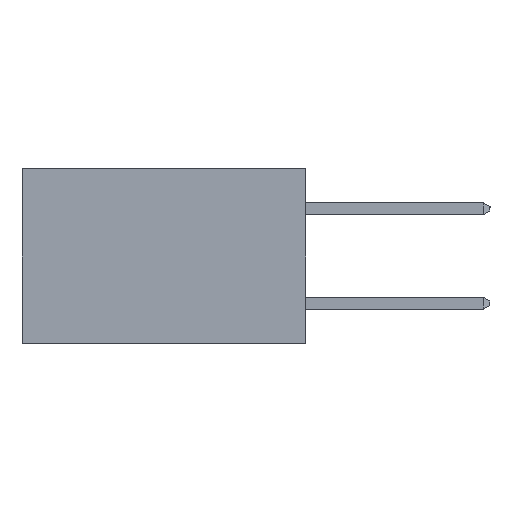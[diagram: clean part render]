
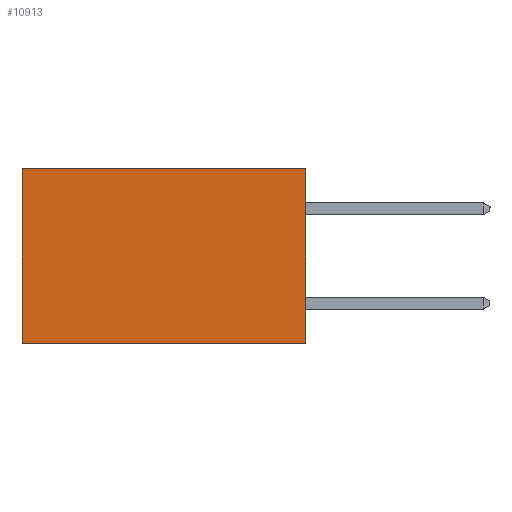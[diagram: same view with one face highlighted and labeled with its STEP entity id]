
A CAD part, left-side view. The second image highlights one B-rep face of the part: STEP entity #10913.
In plain terms, the highlighted planar face has unit normal (-1, 0, 0).
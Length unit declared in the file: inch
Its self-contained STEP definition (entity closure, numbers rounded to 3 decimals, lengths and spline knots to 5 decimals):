
#71 = CARTESIAN_POINT ( 'NONE',  ( 0.2615, 0., 0. ) ) ;
#259 = VERTEX_POINT ( 'NONE', #9011 ) ;
#563 = EDGE_CURVE ( 'NONE', #6719, #9419, #6965, .T. ) ;
#712 = DIRECTION ( 'NONE',  ( 0., 0., -1. ) ) ;
#884 = ORIENTED_EDGE ( 'NONE', *, *, #563, .T. ) ;
#985 = FACE_OUTER_BOUND ( 'NONE', #4562, .T. ) ;
#1040 = CARTESIAN_POINT ( 'NONE',  ( 0.2615, 0., -0.37 ) ) ;
#1124 = VECTOR ( 'NONE', #1654, 39.37008 ) ;
#1567 = LINE ( 'NONE', #5096, #5025 ) ;
#1654 = DIRECTION ( 'NONE',  ( 0., 0., -1. ) ) ;
#1847 = DIRECTION ( 'NONE',  ( 0., 1., 0. ) ) ;
#2847 = EDGE_CURVE ( 'NONE', #9419, #259, #6814, .T. ) ;
#3833 = EDGE_CURVE ( 'NONE', #6719, #6620, #1567, .T. ) ;
#4163 = CARTESIAN_POINT ( 'NONE',  ( 0.2615, 0., -0.37 ) ) ;
#4489 = VECTOR ( 'NONE', #11191, 39.37008 ) ;
#4562 = EDGE_LOOP ( 'NONE', ( #8625, #6116, #5913, #884 ) ) ;
#5025 = VECTOR ( 'NONE', #712, 39.37008 ) ;
#5096 = CARTESIAN_POINT ( 'NONE',  ( 0.2615, 0., -0.37 ) ) ;
#5654 = AXIS2_PLACEMENT_3D ( 'NONE', #1040, #7289, #6247 ) ;
#5769 = VECTOR ( 'NONE', #1847, 39.37008 ) ;
#5913 = ORIENTED_EDGE ( 'NONE', *, *, #3833, .F. ) ;
#6116 = ORIENTED_EDGE ( 'NONE', *, *, #7752, .F. ) ;
#6127 = CARTESIAN_POINT ( 'NONE',  ( 0.2615, 0.6, 0. ) ) ;
#6247 = DIRECTION ( 'NONE',  ( 0., 0., -1. ) ) ;
#6620 = VERTEX_POINT ( 'NONE', #4163 ) ;
#6719 = VERTEX_POINT ( 'NONE', #10519 ) ;
#6814 = LINE ( 'NONE', #8631, #1124 ) ;
#6965 = LINE ( 'NONE', #71, #5769 ) ;
#7289 = DIRECTION ( 'NONE',  ( 1., 0., 0. ) ) ;
#7752 = EDGE_CURVE ( 'NONE', #6620, #259, #8931, .T. ) ;
#8625 = ORIENTED_EDGE ( 'NONE', *, *, #2847, .T. ) ;
#8631 = CARTESIAN_POINT ( 'NONE',  ( 0.2615, 0.6, -0.37 ) ) ;
#8931 = LINE ( 'NONE', #9487, #4489 ) ;
#9011 = CARTESIAN_POINT ( 'NONE',  ( 0.2615, 0.6, -0.37 ) ) ;
#9419 = VERTEX_POINT ( 'NONE', #6127 ) ;
#9487 = CARTESIAN_POINT ( 'NONE',  ( 0.2615, 0., -0.37 ) ) ;
#10519 = CARTESIAN_POINT ( 'NONE',  ( 0.2615, 0., 0. ) ) ;
#10538 = PLANE ( 'NONE',  #5654 ) ;
#10913 = ADVANCED_FACE ( 'NONE', ( #985 ), #10538, .F. ) ;
#11191 = DIRECTION ( 'NONE',  ( 0., 1., 0. ) ) ;
